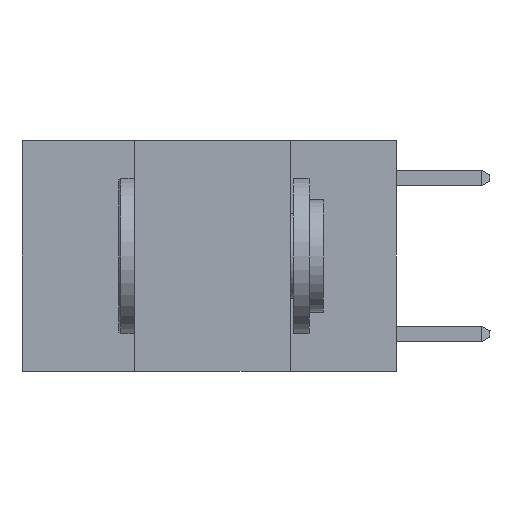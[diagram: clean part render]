
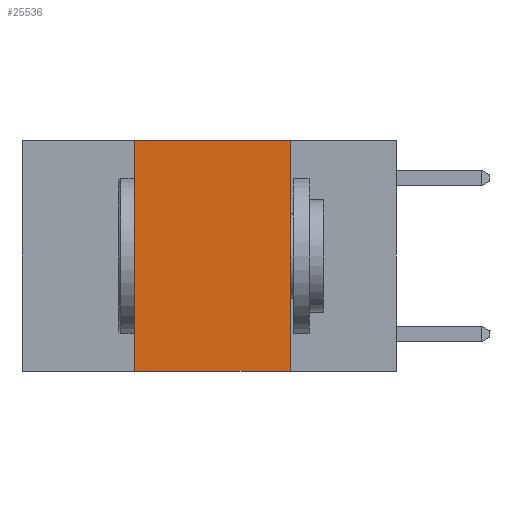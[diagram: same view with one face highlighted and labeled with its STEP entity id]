
A CAD part, left-side view. The second image highlights one B-rep face of the part: STEP entity #25536.
In plain terms, the highlighted planar face has unit normal (-1, 0, 0).
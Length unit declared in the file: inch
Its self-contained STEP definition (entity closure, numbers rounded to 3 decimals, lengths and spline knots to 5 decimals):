
#711 = DIRECTION ( 'NONE',  ( 0., -1., 0. ) ) ;
#1000 = VERTEX_POINT ( 'NONE', #14274 ) ;
#1389 = ORIENTED_EDGE ( 'NONE', *, *, #21542, .F. ) ;
#1679 = EDGE_CURVE ( 'NONE', #13648, #3937, #8017, .T. ) ;
#1722 = VECTOR ( 'NONE', #2566, 39.37008 ) ;
#2566 = DIRECTION ( 'NONE',  ( 0., 0., -1. ) ) ;
#3028 = CARTESIAN_POINT ( 'NONE',  ( 0., 0.17, -0.37 ) ) ;
#3054 = CARTESIAN_POINT ( 'NONE',  ( 0., 0.42, 0. ) ) ;
#3937 = VERTEX_POINT ( 'NONE', #3028 ) ;
#4238 = VECTOR ( 'NONE', #5020, 39.37008 ) ;
#5020 = DIRECTION ( 'NONE',  ( 0., -1., 0. ) ) ;
#5417 = ORIENTED_EDGE ( 'NONE', *, *, #1679, .F. ) ;
#7321 = VERTEX_POINT ( 'NONE', #11721 ) ;
#7672 = ORIENTED_EDGE ( 'NONE', *, *, #15936, .T. ) ;
#8017 = LINE ( 'NONE', #9494, #1722 ) ;
#9494 = CARTESIAN_POINT ( 'NONE',  ( 0., 0.17, 0. ) ) ;
#9997 = PLANE ( 'NONE',  #25452 ) ;
#10523 = LINE ( 'NONE', #25664, #4238 ) ;
#11721 = CARTESIAN_POINT ( 'NONE',  ( 0., 0.42, 0. ) ) ;
#12345 = DIRECTION ( 'NONE',  ( 0., 0., -1. ) ) ;
#12431 = ORIENTED_EDGE ( 'NONE', *, *, #20872, .F. ) ;
#12583 = FACE_OUTER_BOUND ( 'NONE', #16109, .T. ) ;
#13348 = CARTESIAN_POINT ( 'NONE',  ( 0., 0.17, 0. ) ) ;
#13648 = VERTEX_POINT ( 'NONE', #13348 ) ;
#14274 = CARTESIAN_POINT ( 'NONE',  ( 0., 0.42, -0.37 ) ) ;
#14705 = LINE ( 'NONE', #28310, #20026 ) ;
#15507 = LINE ( 'NONE', #3054, #20827 ) ;
#15936 = EDGE_CURVE ( 'NONE', #1000, #3937, #14705, .T. ) ;
#16109 = EDGE_LOOP ( 'NONE', ( #5417, #12431, #1389, #7672 ) ) ;
#16815 = CARTESIAN_POINT ( 'NONE',  ( 0., 0.6, 0. ) ) ;
#19266 = DIRECTION ( 'NONE',  ( 0., 0., 1. ) ) ;
#20026 = VECTOR ( 'NONE', #711, 39.37008 ) ;
#20827 = VECTOR ( 'NONE', #19266, 39.37008 ) ;
#20872 = EDGE_CURVE ( 'NONE', #7321, #13648, #10523, .T. ) ;
#21542 = EDGE_CURVE ( 'NONE', #1000, #7321, #15507, .T. ) ;
#25452 = AXIS2_PLACEMENT_3D ( 'NONE', #16815, #25966, #12345 ) ;
#25536 = ADVANCED_FACE ( 'NONE', ( #12583 ), #9997, .F. ) ;
#25664 = CARTESIAN_POINT ( 'NONE',  ( 0., 0.6, 0. ) ) ;
#25966 = DIRECTION ( 'NONE',  ( 1., 0., 0. ) ) ;
#28310 = CARTESIAN_POINT ( 'NONE',  ( 0., 0.6, -0.37 ) ) ;
